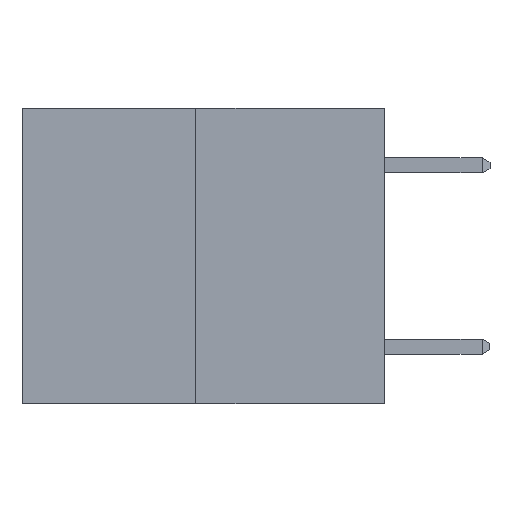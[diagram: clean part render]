
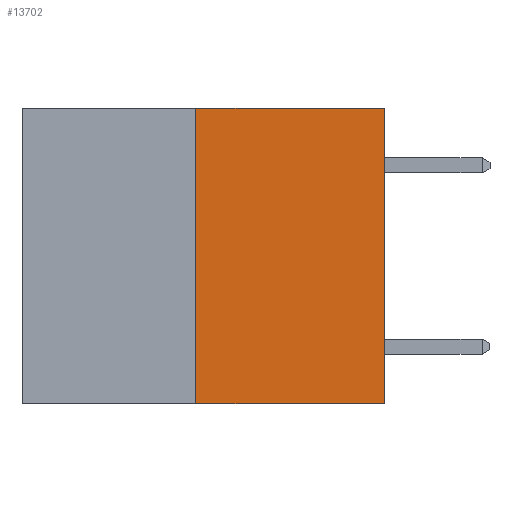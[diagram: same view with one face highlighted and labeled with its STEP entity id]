
A CAD part, left-side view. The second image highlights one B-rep face of the part: STEP entity #13702.
In plain terms, the highlighted planar face has unit normal (-1, 0, 0).
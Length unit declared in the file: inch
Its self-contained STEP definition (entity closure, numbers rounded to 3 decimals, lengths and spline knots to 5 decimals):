
#152 = ORIENTED_EDGE ( 'NONE', *, *, #9965, .T. ) ;
#396 = DIRECTION ( 'NONE',  ( 0., -1., 0. ) ) ;
#1483 = CARTESIAN_POINT ( 'NONE',  ( 0., 0.312, 0. ) ) ;
#1703 = CARTESIAN_POINT ( 'NONE',  ( 0., 0.6, 0. ) ) ;
#1991 = DIRECTION ( 'NONE',  ( 0., 0., 1. ) ) ;
#2114 = FACE_OUTER_BOUND ( 'NONE', #7931, .T. ) ;
#2916 = VECTOR ( 'NONE', #11223, 39.37008 ) ;
#3692 = VECTOR ( 'NONE', #11924, 39.37008 ) ;
#3800 = CARTESIAN_POINT ( 'NONE',  ( 0., 0., -0.49 ) ) ;
#4528 = ORIENTED_EDGE ( 'NONE', *, *, #10191, .F. ) ;
#5286 = ORIENTED_EDGE ( 'NONE', *, *, #6294, .T. ) ;
#5311 = CARTESIAN_POINT ( 'NONE',  ( 0., 0.6, 0. ) ) ;
#5367 = VERTEX_POINT ( 'NONE', #1483 ) ;
#6294 = EDGE_CURVE ( 'NONE', #7350, #6457, #12686, .T. ) ;
#6457 = VERTEX_POINT ( 'NONE', #14594 ) ;
#6856 = VERTEX_POINT ( 'NONE', #12100 ) ;
#7165 = LINE ( 'NONE', #1703, #14433 ) ;
#7350 = VERTEX_POINT ( 'NONE', #3800 ) ;
#7626 = PLANE ( 'NONE',  #9852 ) ;
#7789 = CARTESIAN_POINT ( 'NONE',  ( 0., 0.6, -0.49 ) ) ;
#7931 = EDGE_LOOP ( 'NONE', ( #4528, #152, #5286, #11006 ) ) ;
#9644 = EDGE_CURVE ( 'NONE', #5367, #6457, #7165, .T. ) ;
#9852 = AXIS2_PLACEMENT_3D ( 'NONE', #5311, #13325, #10026 ) ;
#9965 = EDGE_CURVE ( 'NONE', #6856, #7350, #12076, .T. ) ;
#10026 = DIRECTION ( 'NONE',  ( 0., 0., -1. ) ) ;
#10058 = VECTOR ( 'NONE', #1991, 39.37008 ) ;
#10191 = EDGE_CURVE ( 'NONE', #6856, #5367, #11519, .T. ) ;
#11006 = ORIENTED_EDGE ( 'NONE', *, *, #9644, .F. ) ;
#11109 = CARTESIAN_POINT ( 'NONE',  ( 0., 0.312, -0.49 ) ) ;
#11223 = DIRECTION ( 'NONE',  ( 0., -1., 0. ) ) ;
#11519 = LINE ( 'NONE', #11109, #10058 ) ;
#11866 = CARTESIAN_POINT ( 'NONE',  ( 0., 0., 0. ) ) ;
#11924 = DIRECTION ( 'NONE',  ( 0., 0., 1. ) ) ;
#12076 = LINE ( 'NONE', #7789, #2916 ) ;
#12100 = CARTESIAN_POINT ( 'NONE',  ( 0., 0.312, -0.49 ) ) ;
#12686 = LINE ( 'NONE', #11866, #3692 ) ;
#13325 = DIRECTION ( 'NONE',  ( 1., 0., 0. ) ) ;
#13702 = ADVANCED_FACE ( 'NONE', ( #2114 ), #7626, .F. ) ;
#14433 = VECTOR ( 'NONE', #396, 39.37008 ) ;
#14594 = CARTESIAN_POINT ( 'NONE',  ( 0., 0., 0. ) ) ;
